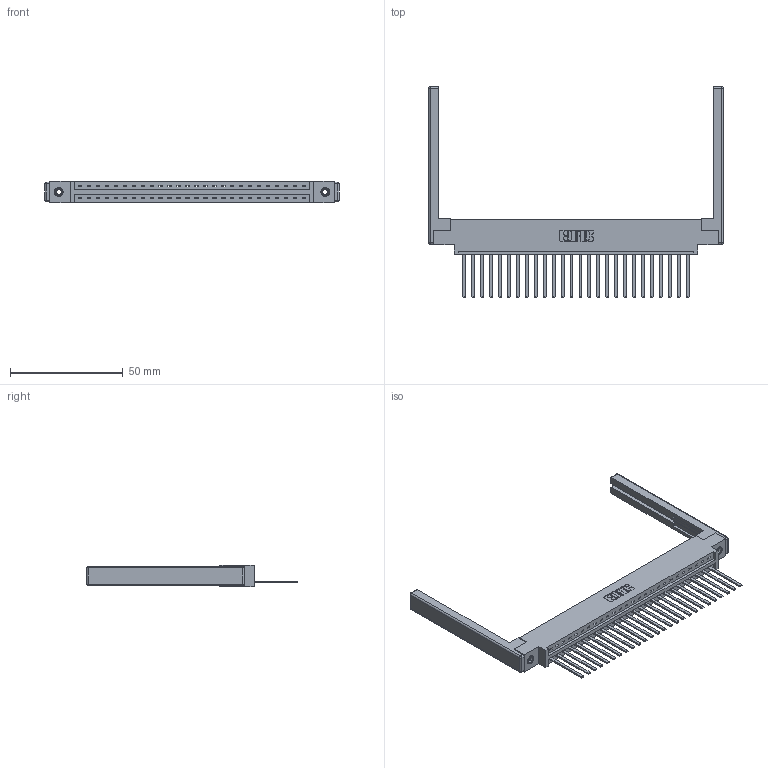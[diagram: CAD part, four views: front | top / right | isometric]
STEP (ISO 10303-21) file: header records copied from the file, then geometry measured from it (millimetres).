
FILE_DESCRIPTION (( 'STEP AP203' ), '1' );
FILE_NAME ('387-026-544-668.STEP', '2019-10-03T13:08:47', ( '' ), ( '' ), 'SwSTEP 2.0', 'SolidWorks 2016', '' );
FILE_SCHEMA (( 'CONFIG_CONTROL_DESIGN' ));
Length unit declared in the file: inch
Products named in the file (5): 345-250-001_345-250-001-102; 337 Part_0.170 Offset - 0.156 Dia-TI; 307-220-068; 387-026-544-668; 345-292-001_345-293-144
Assembly tree (31 placements, depth 2):
  387-026-544-668
    337 Part_0.170 Offset - 0.156 Dia-TI
    345-292-001_345-293-144  x26
    345-250-001_345-250-001-102  x2
    307-220-068  x2
Bounding box: 130.45 x 93.35 x 9.4 mm (x, y, z)
Volume: 17933.1 mm3; surface area: 19084.4 mm2
Topology: 31 solids, 31 shells, 1728 faces, 5133 edges, 3366 vertices
Faces by surface type: plane 1254, cylinder 450, cone 12, sphere 8, torus 4
Entity records: 24104 total; most frequent: CARTESIAN_POINT 4153, ORIENTED_EDGE 4104, DIRECTION 3598, EDGE_CURVE 2052, VECTOR 1878, LINE 1878, VERTEX_POINT 1358, AXIS2_PLACEMENT_3D 860
